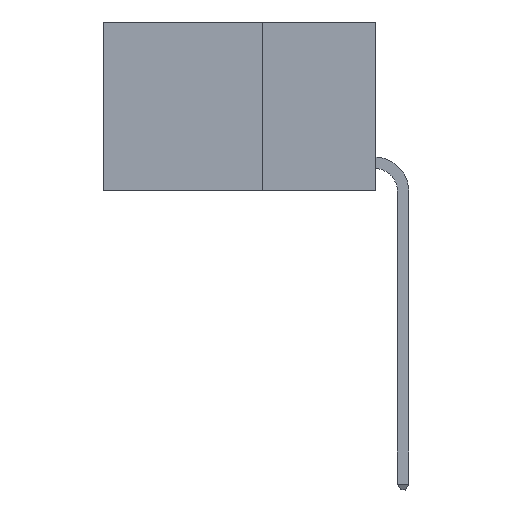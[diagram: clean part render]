
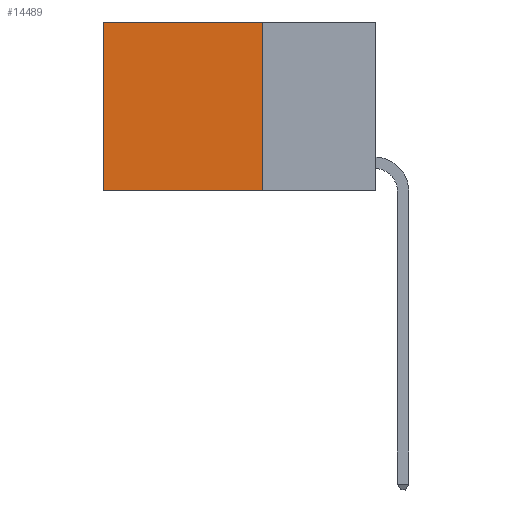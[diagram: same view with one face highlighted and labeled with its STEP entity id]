
A CAD part, left-side view. The second image highlights one B-rep face of the part: STEP entity #14489.
In plain terms, the highlighted planar face has unit normal (-1, 0, 0).
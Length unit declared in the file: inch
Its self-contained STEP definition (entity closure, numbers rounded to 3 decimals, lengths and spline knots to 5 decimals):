
#83 = DIRECTION ( 'NONE',  ( 0., 0., -1. ) ) ;
#430 = EDGE_LOOP ( 'NONE', ( #2535, #1966, #7590, #4968 ) ) ;
#770 = DIRECTION ( 'NONE',  ( 1., 0., 0. ) ) ;
#772 = EDGE_CURVE ( 'NONE', #11321, #4614, #8962, .T. ) ;
#1966 = ORIENTED_EDGE ( 'NONE', *, *, #13063, .F. ) ;
#2043 = VECTOR ( 'NONE', #5561, 39.37008 ) ;
#2341 = CARTESIAN_POINT ( 'NONE',  ( 0.2625, 0.6, 0. ) ) ;
#2535 = ORIENTED_EDGE ( 'NONE', *, *, #4417, .T. ) ;
#2983 = VERTEX_POINT ( 'NONE', #2341 ) ;
#4417 = EDGE_CURVE ( 'NONE', #2983, #9439, #7594, .T. ) ;
#4614 = VERTEX_POINT ( 'NONE', #13304 ) ;
#4968 = ORIENTED_EDGE ( 'NONE', *, *, #15021, .T. ) ;
#5390 = LINE ( 'NONE', #11896, #11764 ) ;
#5561 = DIRECTION ( 'NONE',  ( 0., 0., -1. ) ) ;
#5867 = LINE ( 'NONE', #5987, #12628 ) ;
#5987 = CARTESIAN_POINT ( 'NONE',  ( 0.2625, 0.25, -0.37 ) ) ;
#7590 = ORIENTED_EDGE ( 'NONE', *, *, #772, .F. ) ;
#7594 = LINE ( 'NONE', #15371, #10538 ) ;
#8830 = FACE_OUTER_BOUND ( 'NONE', #430, .T. ) ;
#8962 = LINE ( 'NONE', #15514, #2043 ) ;
#9439 = VERTEX_POINT ( 'NONE', #15301 ) ;
#10538 = VECTOR ( 'NONE', #83, 39.37008 ) ;
#11132 = CARTESIAN_POINT ( 'NONE',  ( 0.2625, 0.25, 0. ) ) ;
#11321 = VERTEX_POINT ( 'NONE', #15606 ) ;
#11764 = VECTOR ( 'NONE', #13173, 39.37008 ) ;
#11896 = CARTESIAN_POINT ( 'NONE',  ( 0.2625, 0.25, 0. ) ) ;
#12402 = PLANE ( 'NONE',  #15277 ) ;
#12628 = VECTOR ( 'NONE', #14851, 39.37008 ) ;
#13063 = EDGE_CURVE ( 'NONE', #4614, #9439, #5867, .T. ) ;
#13173 = DIRECTION ( 'NONE',  ( 0., 1., 0. ) ) ;
#13304 = CARTESIAN_POINT ( 'NONE',  ( 0.2625, 0.25, -0.37 ) ) ;
#13671 = DIRECTION ( 'NONE',  ( 0., 0., -1. ) ) ;
#14489 = ADVANCED_FACE ( 'NONE', ( #8830 ), #12402, .F. ) ;
#14851 = DIRECTION ( 'NONE',  ( 0., 1., 0. ) ) ;
#15021 = EDGE_CURVE ( 'NONE', #11321, #2983, #5390, .T. ) ;
#15277 = AXIS2_PLACEMENT_3D ( 'NONE', #11132, #770, #13671 ) ;
#15301 = CARTESIAN_POINT ( 'NONE',  ( 0.2625, 0.6, -0.37 ) ) ;
#15371 = CARTESIAN_POINT ( 'NONE',  ( 0.2625, 0.6, 0. ) ) ;
#15514 = CARTESIAN_POINT ( 'NONE',  ( 0.2625, 0.25, 0. ) ) ;
#15606 = CARTESIAN_POINT ( 'NONE',  ( 0.2625, 0.25, 0. ) ) ;
